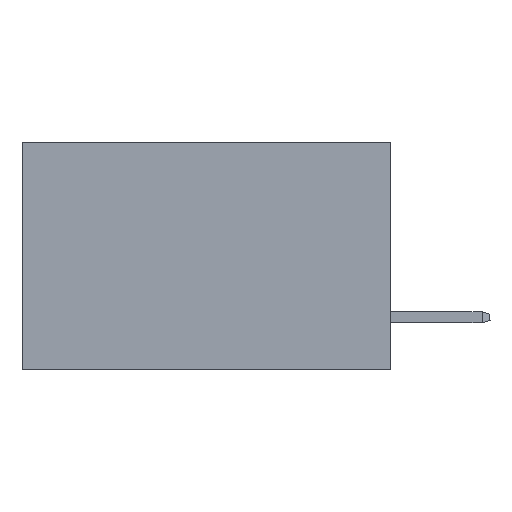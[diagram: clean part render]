
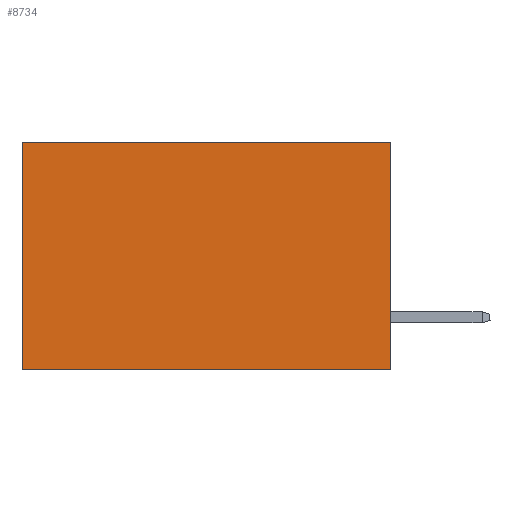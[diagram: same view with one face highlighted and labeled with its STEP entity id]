
A CAD part, left-side view. The second image highlights one B-rep face of the part: STEP entity #8734.
In plain terms, the highlighted planar face has unit normal (-1, 0, 0).
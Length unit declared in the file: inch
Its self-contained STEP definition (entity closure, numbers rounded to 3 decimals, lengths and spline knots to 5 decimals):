
#27 = EDGE_CURVE ( 'NONE', #3941, #4523, #1190, .T. ) ;
#1104 = VECTOR ( 'NONE', #7740, 39.37008 ) ;
#1190 = LINE ( 'NONE', #5468, #7542 ) ;
#1465 = EDGE_CURVE ( 'NONE', #6938, #2742, #6753, .T. ) ;
#2460 = EDGE_CURVE ( 'NONE', #3941, #6938, #10812, .T. ) ;
#2630 = CARTESIAN_POINT ( 'NONE',  ( 0.2875, 0.6, 0. ) ) ;
#2742 = VERTEX_POINT ( 'NONE', #10042 ) ;
#2755 = LINE ( 'NONE', #2630, #4174 ) ;
#2817 = CARTESIAN_POINT ( 'NONE',  ( 0.2875, 0., -0.37 ) ) ;
#2941 = PLANE ( 'NONE',  #10677 ) ;
#3276 = ORIENTED_EDGE ( 'NONE', *, *, #1465, .F. ) ;
#3590 = ORIENTED_EDGE ( 'NONE', *, *, #9654, .T. ) ;
#3941 = VERTEX_POINT ( 'NONE', #4281 ) ;
#4174 = VECTOR ( 'NONE', #7085, 39.37008 ) ;
#4281 = CARTESIAN_POINT ( 'NONE',  ( 0.2875, 0., 0. ) ) ;
#4523 = VERTEX_POINT ( 'NONE', #11582 ) ;
#4667 = DIRECTION ( 'NONE',  ( 0., 1., 0. ) ) ;
#5277 = EDGE_LOOP ( 'NONE', ( #3590, #3276, #9169, #7728 ) ) ;
#5468 = CARTESIAN_POINT ( 'NONE',  ( 0.2875, 0., 0. ) ) ;
#6559 = CARTESIAN_POINT ( 'NONE',  ( 0.2875, 0., 0. ) ) ;
#6670 = DIRECTION ( 'NONE',  ( 0., 0., -1. ) ) ;
#6753 = LINE ( 'NONE', #2817, #9486 ) ;
#6826 = CARTESIAN_POINT ( 'NONE',  ( 0.2875, 0., 0. ) ) ;
#6938 = VERTEX_POINT ( 'NONE', #9121 ) ;
#7085 = DIRECTION ( 'NONE',  ( 0., 0., -1. ) ) ;
#7542 = VECTOR ( 'NONE', #9015, 39.37008 ) ;
#7728 = ORIENTED_EDGE ( 'NONE', *, *, #27, .T. ) ;
#7740 = DIRECTION ( 'NONE',  ( 0., 0., -1. ) ) ;
#8734 = ADVANCED_FACE ( 'NONE', ( #10289 ), #2941, .F. ) ;
#9015 = DIRECTION ( 'NONE',  ( 0., 1., 0. ) ) ;
#9121 = CARTESIAN_POINT ( 'NONE',  ( 0.2875, 0., -0.37 ) ) ;
#9169 = ORIENTED_EDGE ( 'NONE', *, *, #2460, .F. ) ;
#9359 = DIRECTION ( 'NONE',  ( 1., 0., 0. ) ) ;
#9486 = VECTOR ( 'NONE', #4667, 39.37008 ) ;
#9654 = EDGE_CURVE ( 'NONE', #4523, #2742, #2755, .T. ) ;
#10042 = CARTESIAN_POINT ( 'NONE',  ( 0.2875, 0.6, -0.37 ) ) ;
#10289 = FACE_OUTER_BOUND ( 'NONE', #5277, .T. ) ;
#10677 = AXIS2_PLACEMENT_3D ( 'NONE', #6559, #9359, #6670 ) ;
#10812 = LINE ( 'NONE', #6826, #1104 ) ;
#11582 = CARTESIAN_POINT ( 'NONE',  ( 0.2875, 0.6, 0. ) ) ;
